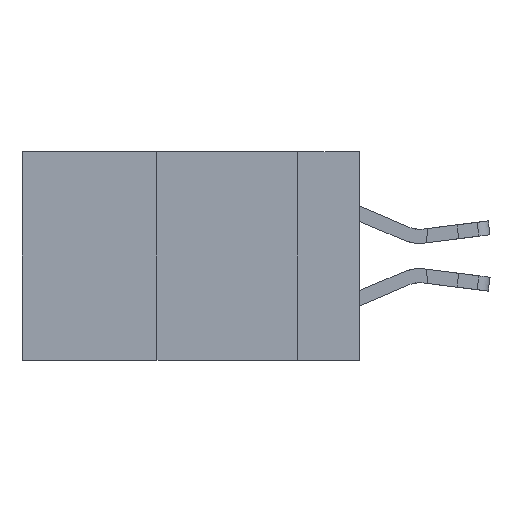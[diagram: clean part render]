
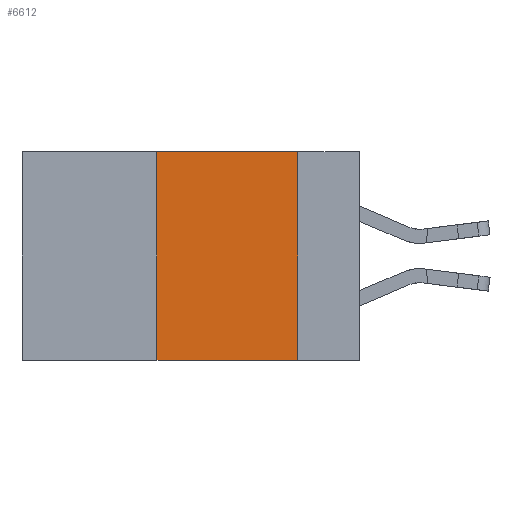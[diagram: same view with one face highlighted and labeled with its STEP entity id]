
A CAD part, left-side view. The second image highlights one B-rep face of the part: STEP entity #6612.
In plain terms, the highlighted planar face has unit normal (-1, 0, 0).
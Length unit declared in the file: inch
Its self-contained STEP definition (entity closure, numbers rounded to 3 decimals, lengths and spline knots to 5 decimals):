
#322 = LINE ( 'NONE', #538, #9946 ) ;
#389 = VERTEX_POINT ( 'NONE', #9259 ) ;
#459 = CARTESIAN_POINT ( 'NONE',  ( 0., 0.6, -0.37 ) ) ;
#538 = CARTESIAN_POINT ( 'NONE',  ( 0., 0.36, 0. ) ) ;
#1958 = LINE ( 'NONE', #7133, #15352 ) ;
#2693 = CARTESIAN_POINT ( 'NONE',  ( 0., 0.11, 0. ) ) ;
#2928 = VECTOR ( 'NONE', #18903, 39.37008 ) ;
#3672 = CARTESIAN_POINT ( 'NONE',  ( 0., 0.36, -0.37 ) ) ;
#3724 = VERTEX_POINT ( 'NONE', #16829 ) ;
#3982 = DIRECTION ( 'NONE',  ( 0., -1., 0. ) ) ;
#4386 = LINE ( 'NONE', #459, #2928 ) ;
#4787 = EDGE_CURVE ( 'NONE', #3724, #389, #13030, .T. ) ;
#4913 = FACE_OUTER_BOUND ( 'NONE', #7500, .T. ) ;
#5188 = DIRECTION ( 'NONE',  ( 0., 0., 1. ) ) ;
#5441 = VERTEX_POINT ( 'NONE', #18167 ) ;
#5656 = DIRECTION ( 'NONE',  ( 0., 0., -1. ) ) ;
#5860 = ORIENTED_EDGE ( 'NONE', *, *, #13704, .F. ) ;
#5991 = PLANE ( 'NONE',  #6434 ) ;
#6434 = AXIS2_PLACEMENT_3D ( 'NONE', #16382, #8471, #15186 ) ;
#6612 = ADVANCED_FACE ( 'NONE', ( #4913 ), #5991, .F. ) ;
#7133 = CARTESIAN_POINT ( 'NONE',  ( 0., 0.6, 0. ) ) ;
#7500 = EDGE_LOOP ( 'NONE', ( #17439, #13904, #5860, #15846 ) ) ;
#7559 = VECTOR ( 'NONE', #5656, 39.37008 ) ;
#7593 = EDGE_CURVE ( 'NONE', #5441, #3724, #1958, .T. ) ;
#8020 = EDGE_CURVE ( 'NONE', #10735, #389, #4386, .T. ) ;
#8471 = DIRECTION ( 'NONE',  ( 1., 0., 0. ) ) ;
#9259 = CARTESIAN_POINT ( 'NONE',  ( 0., 0.11, -0.37 ) ) ;
#9946 = VECTOR ( 'NONE', #5188, 39.37008 ) ;
#10735 = VERTEX_POINT ( 'NONE', #3672 ) ;
#13030 = LINE ( 'NONE', #2693, #7559 ) ;
#13704 = EDGE_CURVE ( 'NONE', #10735, #5441, #322, .T. ) ;
#13904 = ORIENTED_EDGE ( 'NONE', *, *, #7593, .F. ) ;
#15186 = DIRECTION ( 'NONE',  ( 0., 0., -1. ) ) ;
#15352 = VECTOR ( 'NONE', #3982, 39.37008 ) ;
#15846 = ORIENTED_EDGE ( 'NONE', *, *, #8020, .T. ) ;
#16382 = CARTESIAN_POINT ( 'NONE',  ( 0., 0.6, 0. ) ) ;
#16829 = CARTESIAN_POINT ( 'NONE',  ( 0., 0.11, 0. ) ) ;
#17439 = ORIENTED_EDGE ( 'NONE', *, *, #4787, .F. ) ;
#18167 = CARTESIAN_POINT ( 'NONE',  ( 0., 0.36, 0. ) ) ;
#18903 = DIRECTION ( 'NONE',  ( 0., -1., 0. ) ) ;
